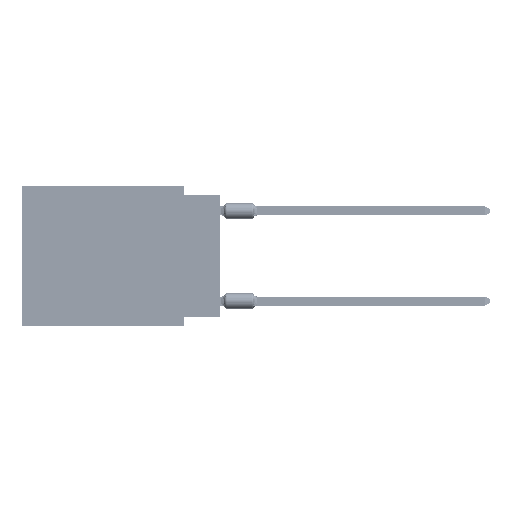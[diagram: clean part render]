
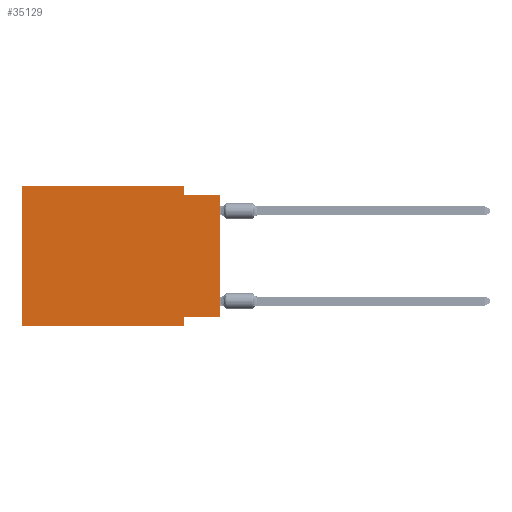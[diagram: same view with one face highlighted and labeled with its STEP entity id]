
A CAD part, left-side view. The second image highlights one B-rep face of the part: STEP entity #35129.
In plain terms, the highlighted planar face has unit normal (-1, 0, 0).
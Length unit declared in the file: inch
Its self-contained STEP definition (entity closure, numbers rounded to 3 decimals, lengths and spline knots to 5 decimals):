
#273 = CARTESIAN_POINT ( 'NONE',  ( 0., 0.55, 0. ) ) ;
#1108 = CARTESIAN_POINT ( 'NONE',  ( 0., 0.1, 0. ) ) ;
#2250 = CARTESIAN_POINT ( 'NONE',  ( 0., 0., -0.365 ) ) ;
#6345 = VECTOR ( 'NONE', #22435, 39.37008 ) ;
#6452 = ORIENTED_EDGE ( 'NONE', *, *, #63690, .F. ) ;
#12320 = LINE ( 'NONE', #41403, #36940 ) ;
#16385 = LINE ( 'NONE', #39438, #6345 ) ;
#17589 = VERTEX_POINT ( 'NONE', #1108 ) ;
#17656 = VERTEX_POINT ( 'NONE', #53617 ) ;
#17824 = CARTESIAN_POINT ( 'NONE',  ( 0., 0.55, 0. ) ) ;
#18961 = VERTEX_POINT ( 'NONE', #72837 ) ;
#20473 = DIRECTION ( 'NONE',  ( 0., 1., 0. ) ) ;
#22435 = DIRECTION ( 'NONE',  ( 0., 0., -1. ) ) ;
#23489 = FACE_OUTER_BOUND ( 'NONE', #23657, .T. ) ;
#23657 = EDGE_LOOP ( 'NONE', ( #72012, #72119, #6452, #50620, #26128, #28656, #51108, #73854 ) ) ;
#25074 = VECTOR ( 'NONE', #60710, 39.37008 ) ;
#26128 = ORIENTED_EDGE ( 'NONE', *, *, #49259, .F. ) ;
#26586 = EDGE_CURVE ( 'NONE', #47531, #17656, #55051, .T. ) ;
#26707 = CARTESIAN_POINT ( 'NONE',  ( 0., 0.1, -0.39 ) ) ;
#28656 = ORIENTED_EDGE ( 'NONE', *, *, #48809, .T. ) ;
#29527 = DIRECTION ( 'NONE',  ( 1., 0., 0. ) ) ;
#29992 = VECTOR ( 'NONE', #65527, 39.37008 ) ;
#33006 = CARTESIAN_POINT ( 'NONE',  ( 0., 0., -0.025 ) ) ;
#34817 = CARTESIAN_POINT ( 'NONE',  ( 0., 0.1, -0.365 ) ) ;
#35129 = ADVANCED_FACE ( 'NONE', ( #23489 ), #46522, .F. ) ;
#36015 = DIRECTION ( 'NONE',  ( 0., -1., 0. ) ) ;
#36940 = VECTOR ( 'NONE', #52386, 39.37008 ) ;
#37553 = CARTESIAN_POINT ( 'NONE',  ( 0., 0.55, 0. ) ) ;
#39438 = CARTESIAN_POINT ( 'NONE',  ( 0., 0.1, 0. ) ) ;
#40863 = DIRECTION ( 'NONE',  ( 0., 0., -1. ) ) ;
#41403 = CARTESIAN_POINT ( 'NONE',  ( 0., 0., 0. ) ) ;
#42627 = EDGE_CURVE ( 'NONE', #74134, #64509, #58337, .T. ) ;
#44636 = LINE ( 'NONE', #67309, #45929 ) ;
#44728 = VERTEX_POINT ( 'NONE', #2250 ) ;
#45929 = VECTOR ( 'NONE', #20473, 39.37008 ) ;
#46351 = DIRECTION ( 'NONE',  ( 0., -1., 0. ) ) ;
#46522 = PLANE ( 'NONE',  #61161 ) ;
#46726 = EDGE_CURVE ( 'NONE', #44728, #64509, #12320, .T. ) ;
#47531 = VERTEX_POINT ( 'NONE', #34817 ) ;
#48809 = EDGE_CURVE ( 'NONE', #65658, #17656, #72379, .T. ) ;
#49259 = EDGE_CURVE ( 'NONE', #65658, #18961, #55322, .T. ) ;
#49761 = DIRECTION ( 'NONE',  ( 0., 0., -1. ) ) ;
#50398 = CARTESIAN_POINT ( 'NONE',  ( 0., 0.55, -0.39 ) ) ;
#50574 = VECTOR ( 'NONE', #46351, 39.37008 ) ;
#50620 = ORIENTED_EDGE ( 'NONE', *, *, #69313, .F. ) ;
#51108 = ORIENTED_EDGE ( 'NONE', *, *, #26586, .F. ) ;
#52386 = DIRECTION ( 'NONE',  ( 0., 0., 1. ) ) ;
#53617 = CARTESIAN_POINT ( 'NONE',  ( 0., 0.1, -0.39 ) ) ;
#55051 = LINE ( 'NONE', #26707, #58125 ) ;
#55322 = LINE ( 'NONE', #37553, #29992 ) ;
#57261 = VECTOR ( 'NONE', #36015, 39.37008 ) ;
#57333 = LINE ( 'NONE', #273, #50574 ) ;
#58125 = VECTOR ( 'NONE', #49761, 39.37008 ) ;
#58337 = LINE ( 'NONE', #58698, #57261 ) ;
#58698 = CARTESIAN_POINT ( 'NONE',  ( 0., 0., -0.025 ) ) ;
#59591 = CARTESIAN_POINT ( 'NONE',  ( 0., 0.55, -0.39 ) ) ;
#59702 = EDGE_CURVE ( 'NONE', #44728, #47531, #44636, .T. ) ;
#60710 = DIRECTION ( 'NONE',  ( 0., -1., 0. ) ) ;
#61161 = AXIS2_PLACEMENT_3D ( 'NONE', #17824, #29527, #40863 ) ;
#63690 = EDGE_CURVE ( 'NONE', #17589, #74134, #16385, .T. ) ;
#64509 = VERTEX_POINT ( 'NONE', #33006 ) ;
#65527 = DIRECTION ( 'NONE',  ( 0., 0., 1. ) ) ;
#65658 = VERTEX_POINT ( 'NONE', #50398 ) ;
#67309 = CARTESIAN_POINT ( 'NONE',  ( 0., 0., -0.365 ) ) ;
#67996 = CARTESIAN_POINT ( 'NONE',  ( 0., 0.1, -0.025 ) ) ;
#69313 = EDGE_CURVE ( 'NONE', #18961, #17589, #57333, .T. ) ;
#72012 = ORIENTED_EDGE ( 'NONE', *, *, #46726, .T. ) ;
#72119 = ORIENTED_EDGE ( 'NONE', *, *, #42627, .F. ) ;
#72379 = LINE ( 'NONE', #59591, #25074 ) ;
#72837 = CARTESIAN_POINT ( 'NONE',  ( 0., 0.55, 0. ) ) ;
#73854 = ORIENTED_EDGE ( 'NONE', *, *, #59702, .F. ) ;
#74134 = VERTEX_POINT ( 'NONE', #67996 ) ;
